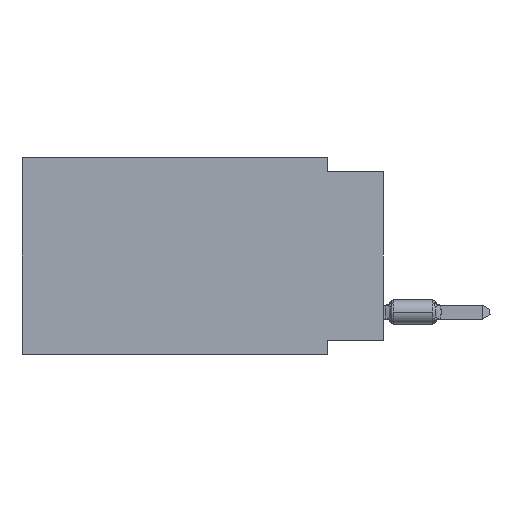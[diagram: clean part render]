
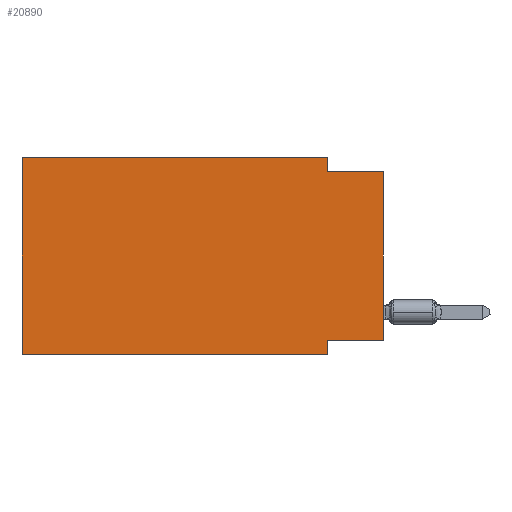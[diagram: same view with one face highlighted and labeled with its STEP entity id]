
A CAD part, left-side view. The second image highlights one B-rep face of the part: STEP entity #20890.
In plain terms, the highlighted planar face has unit normal (-1, 0, 0).
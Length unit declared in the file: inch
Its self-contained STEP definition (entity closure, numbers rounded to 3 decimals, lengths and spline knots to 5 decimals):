
#424 = DIRECTION ( 'NONE',  ( 1., 0., 0. ) ) ;
#791 = LINE ( 'NONE', #59884, #67848 ) ;
#831 = LINE ( 'NONE', #5420, #61118 ) ;
#1319 = EDGE_CURVE ( 'NONE', #67978, #22706, #831, .T. ) ;
#1840 = CARTESIAN_POINT ( 'NONE',  ( 0., 0.1, -0.325 ) ) ;
#2382 = EDGE_CURVE ( 'NONE', #67978, #62961, #59713, .T. ) ;
#3019 = ORIENTED_EDGE ( 'NONE', *, *, #26356, .F. ) ;
#5420 = CARTESIAN_POINT ( 'NONE',  ( 0., 0.645, 0. ) ) ;
#6918 = CARTESIAN_POINT ( 'NONE',  ( 0., 0.645, -0.35 ) ) ;
#7439 = AXIS2_PLACEMENT_3D ( 'NONE', #10944, #424, #16202 ) ;
#9682 = DIRECTION ( 'NONE',  ( 0., -1., 0. ) ) ;
#10944 = CARTESIAN_POINT ( 'NONE',  ( 0., 0.645, 0. ) ) ;
#11908 = CARTESIAN_POINT ( 'NONE',  ( 0., 0.645, 0. ) ) ;
#12017 = LINE ( 'NONE', #31959, #52091 ) ;
#13145 = VERTEX_POINT ( 'NONE', #68249 ) ;
#13308 = DIRECTION ( 'NONE',  ( 0., 1., 0. ) ) ;
#14940 = LINE ( 'NONE', #56567, #20614 ) ;
#16202 = DIRECTION ( 'NONE',  ( 0., 0., -1. ) ) ;
#17383 = ORIENTED_EDGE ( 'NONE', *, *, #37539, .F. ) ;
#18541 = LINE ( 'NONE', #39870, #32629 ) ;
#18838 = EDGE_CURVE ( 'NONE', #34008, #22614, #12017, .T. ) ;
#18890 = DIRECTION ( 'NONE',  ( 0., 0., -1. ) ) ;
#20614 = VECTOR ( 'NONE', #9682, 39.37008 ) ;
#20890 = ADVANCED_FACE ( 'NONE', ( #64098 ), #42098, .F. ) ;
#21513 = DIRECTION ( 'NONE',  ( 0., 0., 1. ) ) ;
#21957 = CARTESIAN_POINT ( 'NONE',  ( 0., 0.645, -0.35 ) ) ;
#22614 = VERTEX_POINT ( 'NONE', #55597 ) ;
#22706 = VERTEX_POINT ( 'NONE', #11908 ) ;
#23180 = DIRECTION ( 'NONE',  ( 0., 0., -1. ) ) ;
#23806 = ORIENTED_EDGE ( 'NONE', *, *, #29440, .F. ) ;
#24427 = DIRECTION ( 'NONE',  ( 0., 0., 1. ) ) ;
#26356 = EDGE_CURVE ( 'NONE', #22706, #13145, #14940, .T. ) ;
#29440 = EDGE_CURVE ( 'NONE', #42618, #39254, #55953, .T. ) ;
#31042 = LINE ( 'NONE', #67047, #57882 ) ;
#31959 = CARTESIAN_POINT ( 'NONE',  ( 0., 0., -0.025 ) ) ;
#32629 = VECTOR ( 'NONE', #18890, 39.37008 ) ;
#32751 = EDGE_CURVE ( 'NONE', #42618, #22614, #31042, .T. ) ;
#34008 = VERTEX_POINT ( 'NONE', #64603 ) ;
#35310 = ORIENTED_EDGE ( 'NONE', *, *, #2382, .T. ) ;
#37539 = EDGE_CURVE ( 'NONE', #39254, #62961, #791, .T. ) ;
#39254 = VERTEX_POINT ( 'NONE', #1840 ) ;
#39542 = ORIENTED_EDGE ( 'NONE', *, *, #1319, .F. ) ;
#39841 = EDGE_LOOP ( 'NONE', ( #55371, #66856, #59573, #3019, #39542, #35310, #17383, #23806 ) ) ;
#39870 = CARTESIAN_POINT ( 'NONE',  ( 0., 0.1, 0. ) ) ;
#42098 = PLANE ( 'NONE',  #7439 ) ;
#42618 = VERTEX_POINT ( 'NONE', #60796 ) ;
#44008 = DIRECTION ( 'NONE',  ( 0., -1., 0. ) ) ;
#52091 = VECTOR ( 'NONE', #54671, 39.37008 ) ;
#53954 = CARTESIAN_POINT ( 'NONE',  ( 0., 0.1, -0.35 ) ) ;
#54671 = DIRECTION ( 'NONE',  ( 0., -1., 0. ) ) ;
#55371 = ORIENTED_EDGE ( 'NONE', *, *, #32751, .T. ) ;
#55597 = CARTESIAN_POINT ( 'NONE',  ( 0., 0., -0.025 ) ) ;
#55953 = LINE ( 'NONE', #63544, #66491 ) ;
#56362 = EDGE_CURVE ( 'NONE', #13145, #34008, #18541, .T. ) ;
#56567 = CARTESIAN_POINT ( 'NONE',  ( 0., 0.645, 0. ) ) ;
#56835 = VECTOR ( 'NONE', #44008, 39.37008 ) ;
#57882 = VECTOR ( 'NONE', #24427, 39.37008 ) ;
#59573 = ORIENTED_EDGE ( 'NONE', *, *, #56362, .F. ) ;
#59713 = LINE ( 'NONE', #6918, #56835 ) ;
#59884 = CARTESIAN_POINT ( 'NONE',  ( 0., 0.1, -0.35 ) ) ;
#60796 = CARTESIAN_POINT ( 'NONE',  ( 0., 0., -0.325 ) ) ;
#61118 = VECTOR ( 'NONE', #21513, 39.37008 ) ;
#62961 = VERTEX_POINT ( 'NONE', #53954 ) ;
#63544 = CARTESIAN_POINT ( 'NONE',  ( 0., 0., -0.325 ) ) ;
#64098 = FACE_OUTER_BOUND ( 'NONE', #39841, .T. ) ;
#64603 = CARTESIAN_POINT ( 'NONE',  ( 0., 0.1, -0.025 ) ) ;
#66491 = VECTOR ( 'NONE', #13308, 39.37008 ) ;
#66856 = ORIENTED_EDGE ( 'NONE', *, *, #18838, .F. ) ;
#67047 = CARTESIAN_POINT ( 'NONE',  ( 0., 0., 0. ) ) ;
#67848 = VECTOR ( 'NONE', #23180, 39.37008 ) ;
#67978 = VERTEX_POINT ( 'NONE', #21957 ) ;
#68249 = CARTESIAN_POINT ( 'NONE',  ( 0., 0.1, 0. ) ) ;
